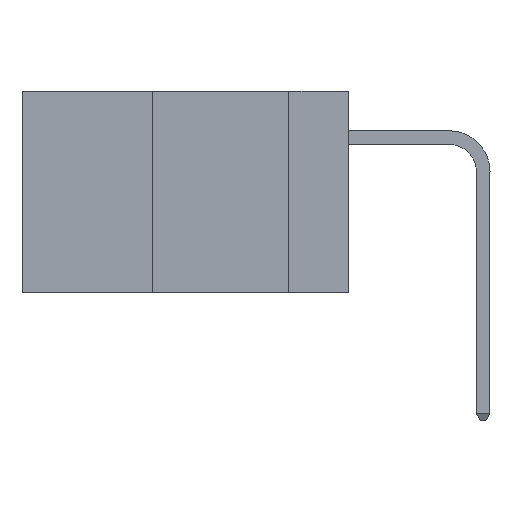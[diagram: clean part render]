
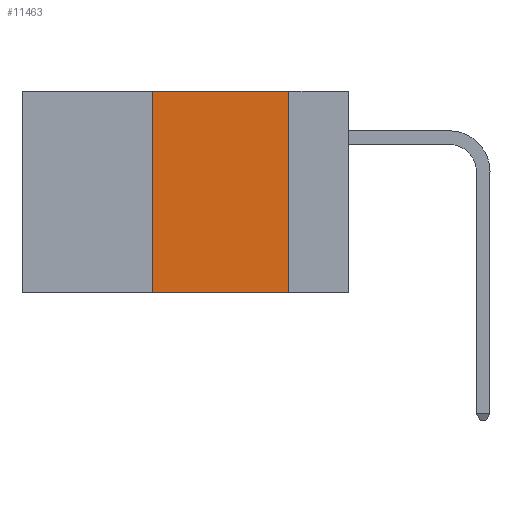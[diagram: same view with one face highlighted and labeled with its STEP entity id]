
A CAD part, left-side view. The second image highlights one B-rep face of the part: STEP entity #11463.
In plain terms, the highlighted planar face has unit normal (-1, 0, 0).
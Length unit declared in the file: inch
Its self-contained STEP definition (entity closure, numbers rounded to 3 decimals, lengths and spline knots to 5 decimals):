
#182 = CARTESIAN_POINT ( 'NONE',  ( 0., 0.36, -0.37 ) ) ;
#420 = CARTESIAN_POINT ( 'NONE',  ( 0., 0.11, 0. ) ) ;
#1683 = VERTEX_POINT ( 'NONE', #182 ) ;
#4080 = VERTEX_POINT ( 'NONE', #19316 ) ;
#5872 = CARTESIAN_POINT ( 'NONE',  ( 0., 0.6, -0.37 ) ) ;
#6749 = EDGE_LOOP ( 'NONE', ( #31745, #14609, #34384, #7168 ) ) ;
#7168 = ORIENTED_EDGE ( 'NONE', *, *, #16182, .T. ) ;
#8009 = CARTESIAN_POINT ( 'NONE',  ( 0., 0.36, 0. ) ) ;
#9318 = LINE ( 'NONE', #27356, #21082 ) ;
#10077 = VERTEX_POINT ( 'NONE', #25786 ) ;
#11286 = DIRECTION ( 'NONE',  ( 0., -1., 0. ) ) ;
#11463 = ADVANCED_FACE ( 'NONE', ( #19396 ), #34344, .F. ) ;
#12548 = VERTEX_POINT ( 'NONE', #8009 ) ;
#14494 = AXIS2_PLACEMENT_3D ( 'NONE', #31769, #15730, #34463 ) ;
#14609 = ORIENTED_EDGE ( 'NONE', *, *, #18200, .F. ) ;
#15655 = LINE ( 'NONE', #5872, #21931 ) ;
#15730 = DIRECTION ( 'NONE',  ( 1., 0., 0. ) ) ;
#16182 = EDGE_CURVE ( 'NONE', #1683, #4080, #15655, .T. ) ;
#18200 = EDGE_CURVE ( 'NONE', #12548, #10077, #32253, .T. ) ;
#19316 = CARTESIAN_POINT ( 'NONE',  ( 0., 0.11, -0.37 ) ) ;
#19396 = FACE_OUTER_BOUND ( 'NONE', #6749, .T. ) ;
#19683 = VECTOR ( 'NONE', #29388, 39.37008 ) ;
#20132 = VECTOR ( 'NONE', #21894, 39.37008 ) ;
#21082 = VECTOR ( 'NONE', #30035, 39.37008 ) ;
#21894 = DIRECTION ( 'NONE',  ( 0., 0., -1. ) ) ;
#21931 = VECTOR ( 'NONE', #11286, 39.37008 ) ;
#22401 = EDGE_CURVE ( 'NONE', #1683, #12548, #9318, .T. ) ;
#25786 = CARTESIAN_POINT ( 'NONE',  ( 0., 0.11, 0. ) ) ;
#26698 = CARTESIAN_POINT ( 'NONE',  ( 0., 0.6, 0. ) ) ;
#27356 = CARTESIAN_POINT ( 'NONE',  ( 0., 0.36, 0. ) ) ;
#28261 = EDGE_CURVE ( 'NONE', #10077, #4080, #28945, .T. ) ;
#28945 = LINE ( 'NONE', #420, #20132 ) ;
#29388 = DIRECTION ( 'NONE',  ( 0., -1., 0. ) ) ;
#30035 = DIRECTION ( 'NONE',  ( 0., 0., 1. ) ) ;
#31745 = ORIENTED_EDGE ( 'NONE', *, *, #28261, .F. ) ;
#31769 = CARTESIAN_POINT ( 'NONE',  ( 0., 0.6, 0. ) ) ;
#32253 = LINE ( 'NONE', #26698, #19683 ) ;
#34344 = PLANE ( 'NONE',  #14494 ) ;
#34384 = ORIENTED_EDGE ( 'NONE', *, *, #22401, .F. ) ;
#34463 = DIRECTION ( 'NONE',  ( 0., 0., -1. ) ) ;
